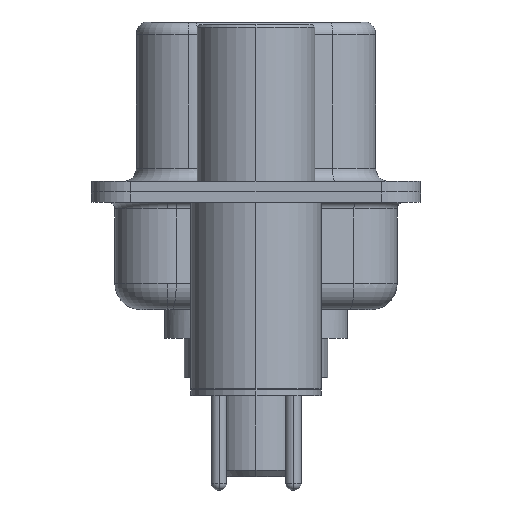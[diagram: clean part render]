
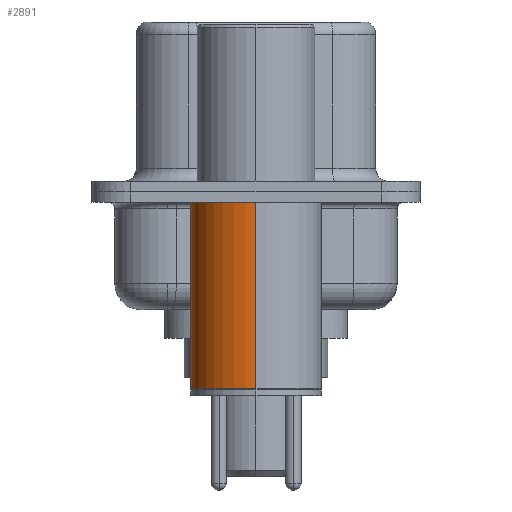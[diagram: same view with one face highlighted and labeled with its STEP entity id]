
A CAD part, left-side view. The second image highlights one B-rep face of the part: STEP entity #2891.
In plain terms, the highlighted cylindrical face has radius 2.5 mm (diameter 5 mm), a partial arc.
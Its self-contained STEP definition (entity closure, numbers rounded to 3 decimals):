
#414 = VECTOR ( 'NONE', #10461, 1000. ) ;
#948 = VECTOR ( 'NONE', #17976, 1000. ) ;
#1050 = EDGE_CURVE ( 'NONE', #16803, #10321, #14639, .T. ) ;
#2467 = CYLINDRICAL_SURFACE ( 'NONE', #7557, 2.5 ) ;
#2891 = ADVANCED_FACE ( 'NONE', ( #19756 ), #2467, .T. ) ;
#5434 = LINE ( 'NONE', #8729, #414 ) ;
#5917 = CARTESIAN_POINT ( 'NONE',  ( 0., 0., -7.525 ) ) ;
#6656 = CARTESIAN_POINT ( 'NONE',  ( -2.5, 0., 0.581 ) ) ;
#7540 = DIRECTION ( 'NONE',  ( 1., 0., 0. ) ) ;
#7557 = AXIS2_PLACEMENT_3D ( 'NONE', #15918, #20196, #9624 ) ;
#7658 = VERTEX_POINT ( 'NONE', #18754 ) ;
#8729 = CARTESIAN_POINT ( 'NONE',  ( 2.5, 0., 0.581 ) ) ;
#9010 = ORIENTED_EDGE ( 'NONE', *, *, #1050, .F. ) ;
#9053 = VERTEX_POINT ( 'NONE', #14174 ) ;
#9116 = ORIENTED_EDGE ( 'NONE', *, *, #10462, .T. ) ;
#9530 = ORIENTED_EDGE ( 'NONE', *, *, #13708, .T. ) ;
#9624 = DIRECTION ( 'NONE',  ( 1., 0., 0. ) ) ;
#9644 = ORIENTED_EDGE ( 'NONE', *, *, #18956, .F. ) ;
#10321 = VERTEX_POINT ( 'NONE', #12203 ) ;
#10461 = DIRECTION ( 'NONE',  ( 0., 0., 1. ) ) ;
#10462 = EDGE_CURVE ( 'NONE', #9053, #7658, #18636, .T. ) ;
#12203 = CARTESIAN_POINT ( 'NONE',  ( -2.5, 0., -0.4 ) ) ;
#13708 = EDGE_CURVE ( 'NONE', #7658, #10321, #14153, .T. ) ;
#14153 = LINE ( 'NONE', #6656, #948 ) ;
#14174 = CARTESIAN_POINT ( 'NONE',  ( 2.5, 0., -7.525 ) ) ;
#14639 = CIRCLE ( 'NONE', #18746, 2.5 ) ;
#15918 = CARTESIAN_POINT ( 'NONE',  ( 0., 0., 0.581 ) ) ;
#16154 = DIRECTION ( 'NONE',  ( 0., 0., 1. ) ) ;
#16266 = AXIS2_PLACEMENT_3D ( 'NONE', #5917, #17261, #7540 ) ;
#16803 = VERTEX_POINT ( 'NONE', #17367 ) ;
#16960 = EDGE_LOOP ( 'NONE', ( #9116, #9530, #9010, #9644 ) ) ;
#17261 = DIRECTION ( 'NONE',  ( 0., 0., 1. ) ) ;
#17367 = CARTESIAN_POINT ( 'NONE',  ( 2.5, 0., -0.4 ) ) ;
#17666 = CARTESIAN_POINT ( 'NONE',  ( 0., 0., -0.4 ) ) ;
#17903 = DIRECTION ( 'NONE',  ( 1., 0., 0. ) ) ;
#17976 = DIRECTION ( 'NONE',  ( 0., 0., 1. ) ) ;
#18636 = CIRCLE ( 'NONE', #16266, 2.5 ) ;
#18746 = AXIS2_PLACEMENT_3D ( 'NONE', #17666, #16154, #17903 ) ;
#18754 = CARTESIAN_POINT ( 'NONE',  ( -2.5, 0., -7.525 ) ) ;
#18956 = EDGE_CURVE ( 'NONE', #9053, #16803, #5434, .T. ) ;
#19756 = FACE_OUTER_BOUND ( 'NONE', #16960, .T. ) ;
#20196 = DIRECTION ( 'NONE',  ( 0., 0., 1. ) ) ;
